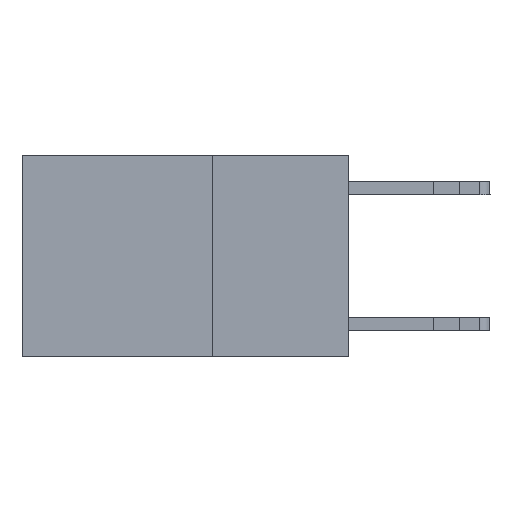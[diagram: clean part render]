
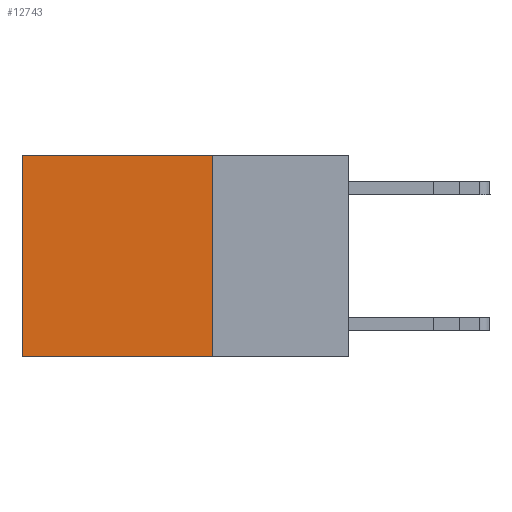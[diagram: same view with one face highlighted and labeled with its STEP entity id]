
A CAD part, left-side view. The second image highlights one B-rep face of the part: STEP entity #12743.
In plain terms, the highlighted planar face has unit normal (-1, 0, 0).
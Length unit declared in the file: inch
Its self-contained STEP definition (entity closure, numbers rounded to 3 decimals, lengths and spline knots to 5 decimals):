
#125 = LINE ( 'NONE', #8927, #11107 ) ;
#701 = VECTOR ( 'NONE', #8700, 39.37008 ) ;
#760 = DIRECTION ( 'NONE',  ( 0., 0., -1. ) ) ;
#1327 = CARTESIAN_POINT ( 'NONE',  ( 0.2625, 0.6, 0. ) ) ;
#1585 = VERTEX_POINT ( 'NONE', #4409 ) ;
#1716 = DIRECTION ( 'NONE',  ( 0., 0., -1. ) ) ;
#2201 = ORIENTED_EDGE ( 'NONE', *, *, #4755, .F. ) ;
#3381 = LINE ( 'NONE', #8528, #13795 ) ;
#4409 = CARTESIAN_POINT ( 'NONE',  ( 0.2625, 0.25, 0. ) ) ;
#4538 = CARTESIAN_POINT ( 'NONE',  ( 0.2625, 0.25, -0.37 ) ) ;
#4550 = ORIENTED_EDGE ( 'NONE', *, *, #10427, .T. ) ;
#4631 = ORIENTED_EDGE ( 'NONE', *, *, #6590, .F. ) ;
#4755 = EDGE_CURVE ( 'NONE', #6196, #5121, #12672, .T. ) ;
#4951 = FACE_OUTER_BOUND ( 'NONE', #6211, .T. ) ;
#5121 = VERTEX_POINT ( 'NONE', #13680 ) ;
#5680 = DIRECTION ( 'NONE',  ( 0., 1., 0. ) ) ;
#5847 = AXIS2_PLACEMENT_3D ( 'NONE', #9809, #7644, #760 ) ;
#6196 = VERTEX_POINT ( 'NONE', #4538 ) ;
#6211 = EDGE_LOOP ( 'NONE', ( #10071, #2201, #4631, #4550 ) ) ;
#6590 = EDGE_CURVE ( 'NONE', #1585, #6196, #3381, .T. ) ;
#7644 = DIRECTION ( 'NONE',  ( 1., 0., 0. ) ) ;
#8180 = DIRECTION ( 'NONE',  ( 0., 0., -1. ) ) ;
#8512 = VERTEX_POINT ( 'NONE', #12064 ) ;
#8528 = CARTESIAN_POINT ( 'NONE',  ( 0.2625, 0.25, 0. ) ) ;
#8700 = DIRECTION ( 'NONE',  ( 0., 1., 0. ) ) ;
#8927 = CARTESIAN_POINT ( 'NONE',  ( 0.2625, 0.25, 0. ) ) ;
#9809 = CARTESIAN_POINT ( 'NONE',  ( 0.2625, 0.25, 0. ) ) ;
#10071 = ORIENTED_EDGE ( 'NONE', *, *, #12475, .T. ) ;
#10427 = EDGE_CURVE ( 'NONE', #1585, #8512, #125, .T. ) ;
#11107 = VECTOR ( 'NONE', #5680, 39.37008 ) ;
#11420 = LINE ( 'NONE', #1327, #14322 ) ;
#12005 = PLANE ( 'NONE',  #5847 ) ;
#12064 = CARTESIAN_POINT ( 'NONE',  ( 0.2625, 0.6, 0. ) ) ;
#12475 = EDGE_CURVE ( 'NONE', #8512, #5121, #11420, .T. ) ;
#12672 = LINE ( 'NONE', #13050, #701 ) ;
#12743 = ADVANCED_FACE ( 'NONE', ( #4951 ), #12005, .F. ) ;
#13050 = CARTESIAN_POINT ( 'NONE',  ( 0.2625, 0.25, -0.37 ) ) ;
#13680 = CARTESIAN_POINT ( 'NONE',  ( 0.2625, 0.6, -0.37 ) ) ;
#13795 = VECTOR ( 'NONE', #1716, 39.37008 ) ;
#14322 = VECTOR ( 'NONE', #8180, 39.37008 ) ;
